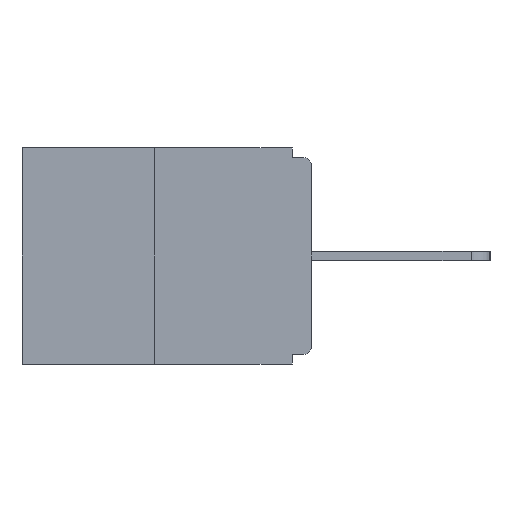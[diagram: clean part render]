
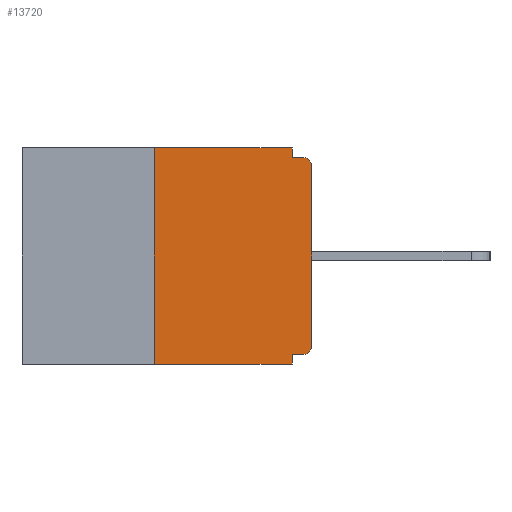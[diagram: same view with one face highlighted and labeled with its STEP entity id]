
A CAD part, left-side view. The second image highlights one B-rep face of the part: STEP entity #13720.
In plain terms, the highlighted planar face has unit normal (-1, 0, 0).
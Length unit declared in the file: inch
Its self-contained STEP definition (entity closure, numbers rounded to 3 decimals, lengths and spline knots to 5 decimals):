
#118 = LINE ( 'NONE', #3823, #15872 ) ;
#518 = LINE ( 'NONE', #11756, #15761 ) ;
#613 = LINE ( 'NONE', #9335, #16660 ) ;
#663 = DIRECTION ( 'NONE',  ( 0., 0., -1. ) ) ;
#759 = CARTESIAN_POINT ( 'NONE',  ( 0., 0., -0.313 ) ) ;
#808 = VERTEX_POINT ( 'NONE', #11397 ) ;
#1093 = EDGE_CURVE ( 'NONE', #16882, #21388, #2482, .T. ) ;
#1312 = AXIS2_PLACEMENT_3D ( 'NONE', #1574, #7178, #20137 ) ;
#1574 = CARTESIAN_POINT ( 'NONE',  ( 0., 0.015, -0.03 ) ) ;
#1660 = CARTESIAN_POINT ( 'NONE',  ( 0., 0.015, -0.313 ) ) ;
#2077 = EDGE_CURVE ( 'NONE', #14227, #808, #518, .T. ) ;
#2429 = EDGE_CURVE ( 'NONE', #11854, #21388, #613, .T. ) ;
#2430 = DIRECTION ( 'NONE',  ( 0., -1., 0. ) ) ;
#2482 = CIRCLE ( 'NONE', #1312, 0.015 ) ;
#2899 = EDGE_CURVE ( 'NONE', #7550, #16882, #118, .T. ) ;
#2932 = PLANE ( 'NONE',  #15149 ) ;
#3286 = VECTOR ( 'NONE', #10499, 39.37008 ) ;
#3756 = VECTOR ( 'NONE', #12870, 39.37008 ) ;
#3823 = CARTESIAN_POINT ( 'NONE',  ( 0., 0., 0. ) ) ;
#4078 = DIRECTION ( 'NONE',  ( 0., -1., 0. ) ) ;
#4246 = FACE_OUTER_BOUND ( 'NONE', #5827, .T. ) ;
#5031 = ORIENTED_EDGE ( 'NONE', *, *, #12934, .F. ) ;
#5190 = ORIENTED_EDGE ( 'NONE', *, *, #1093, .T. ) ;
#5456 = VECTOR ( 'NONE', #21700, 39.37008 ) ;
#5593 = CARTESIAN_POINT ( 'NONE',  ( 0., 0.015, -0.328 ) ) ;
#5827 = EDGE_LOOP ( 'NONE', ( #5031, #13715, #10063, #6072, #11682, #15148, #15415, #5190, #19922, #17453 ) ) ;
#5870 = CARTESIAN_POINT ( 'NONE',  ( 0., 0., -0.03 ) ) ;
#5942 = CARTESIAN_POINT ( 'NONE',  ( 0., 0.015, -0.015 ) ) ;
#6072 = ORIENTED_EDGE ( 'NONE', *, *, #14818, .F. ) ;
#6077 = VERTEX_POINT ( 'NONE', #10437 ) ;
#6367 = VECTOR ( 'NONE', #14446, 39.37008 ) ;
#7135 = CARTESIAN_POINT ( 'NONE',  ( 0., 0.031, 0. ) ) ;
#7178 = DIRECTION ( 'NONE',  ( -1., 0., 0. ) ) ;
#7550 = VERTEX_POINT ( 'NONE', #759 ) ;
#8022 = EDGE_CURVE ( 'NONE', #14227, #6077, #19901, .T. ) ;
#8059 = DIRECTION ( 'NONE',  ( 1., 0., 0. ) ) ;
#8117 = CARTESIAN_POINT ( 'NONE',  ( 0., 0.031, 0. ) ) ;
#8715 = DIRECTION ( 'NONE',  ( 0., 1., 0. ) ) ;
#9335 = CARTESIAN_POINT ( 'NONE',  ( 0., 0., -0.015 ) ) ;
#9656 = EDGE_CURVE ( 'NONE', #20029, #7550, #13156, .T. ) ;
#9682 = EDGE_CURVE ( 'NONE', #20029, #9995, #17933, .T. ) ;
#9995 = VERTEX_POINT ( 'NONE', #17083 ) ;
#10063 = ORIENTED_EDGE ( 'NONE', *, *, #2077, .T. ) ;
#10297 = CARTESIAN_POINT ( 'NONE',  ( 0., 0.46, 0. ) ) ;
#10395 = DIRECTION ( 'NONE',  ( -1., 0., 0. ) ) ;
#10437 = CARTESIAN_POINT ( 'NONE',  ( 0., 0.25, 0. ) ) ;
#10499 = DIRECTION ( 'NONE',  ( 0., -1., 0. ) ) ;
#10509 = DIRECTION ( 'NONE',  ( 0., 0., -1. ) ) ;
#11110 = DIRECTION ( 'NONE',  ( 0., 0., 1. ) ) ;
#11397 = CARTESIAN_POINT ( 'NONE',  ( 0., 0.031, -0.343 ) ) ;
#11682 = ORIENTED_EDGE ( 'NONE', *, *, #9682, .F. ) ;
#11756 = CARTESIAN_POINT ( 'NONE',  ( 0., 0.46, -0.343 ) ) ;
#11854 = VERTEX_POINT ( 'NONE', #22698 ) ;
#12870 = DIRECTION ( 'NONE',  ( 0., 0., -1. ) ) ;
#12891 = VERTEX_POINT ( 'NONE', #8117 ) ;
#12934 = EDGE_CURVE ( 'NONE', #6077, #12891, #19622, .T. ) ;
#12990 = CARTESIAN_POINT ( 'NONE',  ( 0., 0.031, -0.343 ) ) ;
#13156 = CIRCLE ( 'NONE', #18114, 0.015 ) ;
#13715 = ORIENTED_EDGE ( 'NONE', *, *, #8022, .F. ) ;
#13720 = ADVANCED_FACE ( 'NONE', ( #4246 ), #2932, .F. ) ;
#14209 = CARTESIAN_POINT ( 'NONE',  ( 0., 0., -0.328 ) ) ;
#14227 = VERTEX_POINT ( 'NONE', #20226 ) ;
#14446 = DIRECTION ( 'NONE',  ( 0., 0., -1. ) ) ;
#14818 = EDGE_CURVE ( 'NONE', #9995, #808, #20313, .T. ) ;
#15148 = ORIENTED_EDGE ( 'NONE', *, *, #9656, .T. ) ;
#15149 = AXIS2_PLACEMENT_3D ( 'NONE', #18841, #8059, #663 ) ;
#15415 = ORIENTED_EDGE ( 'NONE', *, *, #2899, .T. ) ;
#15761 = VECTOR ( 'NONE', #2430, 39.37008 ) ;
#15872 = VECTOR ( 'NONE', #11110, 39.37008 ) ;
#16660 = VECTOR ( 'NONE', #4078, 39.37008 ) ;
#16882 = VERTEX_POINT ( 'NONE', #5870 ) ;
#17083 = CARTESIAN_POINT ( 'NONE',  ( 0., 0.031, -0.328 ) ) ;
#17453 = ORIENTED_EDGE ( 'NONE', *, *, #21150, .F. ) ;
#17933 = LINE ( 'NONE', #14209, #22760 ) ;
#18114 = AXIS2_PLACEMENT_3D ( 'NONE', #1660, #10395, #10509 ) ;
#18285 = LINE ( 'NONE', #7135, #6367 ) ;
#18841 = CARTESIAN_POINT ( 'NONE',  ( 0., 0.46, 0. ) ) ;
#19622 = LINE ( 'NONE', #10297, #3286 ) ;
#19655 = CARTESIAN_POINT ( 'NONE',  ( 0., 0.25, 0. ) ) ;
#19901 = LINE ( 'NONE', #19655, #5456 ) ;
#19922 = ORIENTED_EDGE ( 'NONE', *, *, #2429, .F. ) ;
#20029 = VERTEX_POINT ( 'NONE', #5593 ) ;
#20137 = DIRECTION ( 'NONE',  ( 0., 0., -1. ) ) ;
#20226 = CARTESIAN_POINT ( 'NONE',  ( 0., 0.25, -0.343 ) ) ;
#20313 = LINE ( 'NONE', #12990, #3756 ) ;
#21150 = EDGE_CURVE ( 'NONE', #12891, #11854, #18285, .T. ) ;
#21388 = VERTEX_POINT ( 'NONE', #5942 ) ;
#21700 = DIRECTION ( 'NONE',  ( 0., 0., 1. ) ) ;
#22698 = CARTESIAN_POINT ( 'NONE',  ( 0., 0.031, -0.015 ) ) ;
#22760 = VECTOR ( 'NONE', #8715, 39.37008 ) ;
